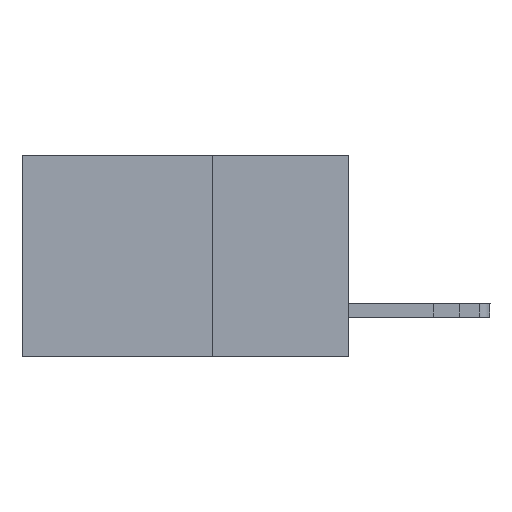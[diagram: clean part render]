
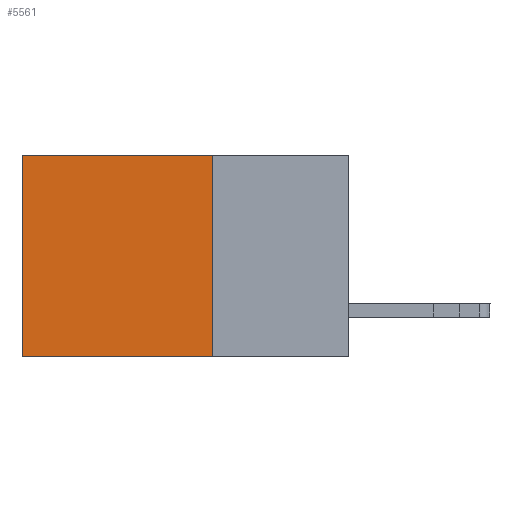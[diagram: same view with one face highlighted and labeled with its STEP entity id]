
A CAD part, left-side view. The second image highlights one B-rep face of the part: STEP entity #5561.
In plain terms, the highlighted planar face has unit normal (-1, 0, 0).
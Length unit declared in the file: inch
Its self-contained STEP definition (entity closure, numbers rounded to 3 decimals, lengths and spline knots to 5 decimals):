
#9 = LINE ( 'NONE', #5013, #12480 ) ;
#283 = CARTESIAN_POINT ( 'NONE',  ( 0.298, 0.25, 0. ) ) ;
#321 = ORIENTED_EDGE ( 'NONE', *, *, #5869, .T. ) ;
#804 = EDGE_LOOP ( 'NONE', ( #9669, #4624, #3980, #321 ) ) ;
#1176 = DIRECTION ( 'NONE',  ( 0., 1., 0. ) ) ;
#1298 = CARTESIAN_POINT ( 'NONE',  ( 0.298, 0.25, -0.37 ) ) ;
#1466 = VECTOR ( 'NONE', #1176, 39.37008 ) ;
#1958 = CARTESIAN_POINT ( 'NONE',  ( 0.298, 0.6, 0. ) ) ;
#2908 = VERTEX_POINT ( 'NONE', #3437 ) ;
#3437 = CARTESIAN_POINT ( 'NONE',  ( 0.298, 0.6, -0.37 ) ) ;
#3618 = AXIS2_PLACEMENT_3D ( 'NONE', #11805, #12708, #9538 ) ;
#3980 = ORIENTED_EDGE ( 'NONE', *, *, #12127, .F. ) ;
#4073 = DIRECTION ( 'NONE',  ( 0., 0., -1. ) ) ;
#4624 = ORIENTED_EDGE ( 'NONE', *, *, #7912, .F. ) ;
#5013 = CARTESIAN_POINT ( 'NONE',  ( 0.298, 0.6, 0. ) ) ;
#5323 = CARTESIAN_POINT ( 'NONE',  ( 0.298, 0.25, -0.37 ) ) ;
#5561 = ADVANCED_FACE ( 'NONE', ( #6479 ), #7114, .F. ) ;
#5869 = EDGE_CURVE ( 'NONE', #9994, #11607, #11768, .T. ) ;
#6479 = FACE_OUTER_BOUND ( 'NONE', #804, .T. ) ;
#7114 = PLANE ( 'NONE',  #3618 ) ;
#7873 = DIRECTION ( 'NONE',  ( 0., 0., -1. ) ) ;
#7912 = EDGE_CURVE ( 'NONE', #8539, #2908, #13042, .T. ) ;
#8539 = VERTEX_POINT ( 'NONE', #5323 ) ;
#8943 = VECTOR ( 'NONE', #7873, 39.37008 ) ;
#8959 = CARTESIAN_POINT ( 'NONE',  ( 0.298, 0.25, 0. ) ) ;
#9284 = LINE ( 'NONE', #283, #8943 ) ;
#9538 = DIRECTION ( 'NONE',  ( 0., 0., -1. ) ) ;
#9669 = ORIENTED_EDGE ( 'NONE', *, *, #9735, .T. ) ;
#9735 = EDGE_CURVE ( 'NONE', #11607, #2908, #9, .T. ) ;
#9901 = CARTESIAN_POINT ( 'NONE',  ( 0.298, 0.25, 0. ) ) ;
#9994 = VERTEX_POINT ( 'NONE', #8959 ) ;
#10108 = DIRECTION ( 'NONE',  ( 0., 1., 0. ) ) ;
#10525 = VECTOR ( 'NONE', #10108, 39.37008 ) ;
#11607 = VERTEX_POINT ( 'NONE', #1958 ) ;
#11768 = LINE ( 'NONE', #9901, #1466 ) ;
#11805 = CARTESIAN_POINT ( 'NONE',  ( 0.298, 0.25, 0. ) ) ;
#12127 = EDGE_CURVE ( 'NONE', #9994, #8539, #9284, .T. ) ;
#12480 = VECTOR ( 'NONE', #4073, 39.37008 ) ;
#12708 = DIRECTION ( 'NONE',  ( 1., 0., 0. ) ) ;
#13042 = LINE ( 'NONE', #1298, #10525 ) ;
